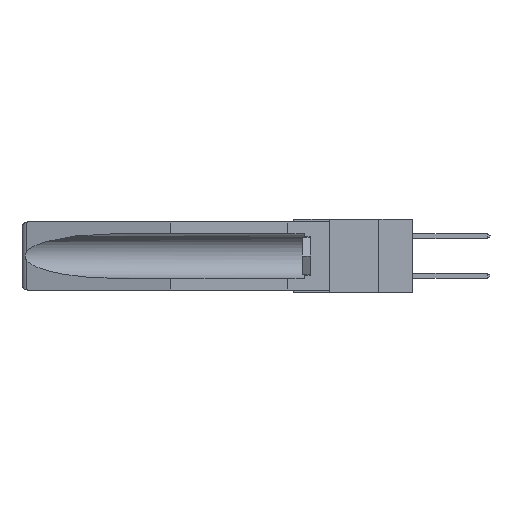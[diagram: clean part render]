
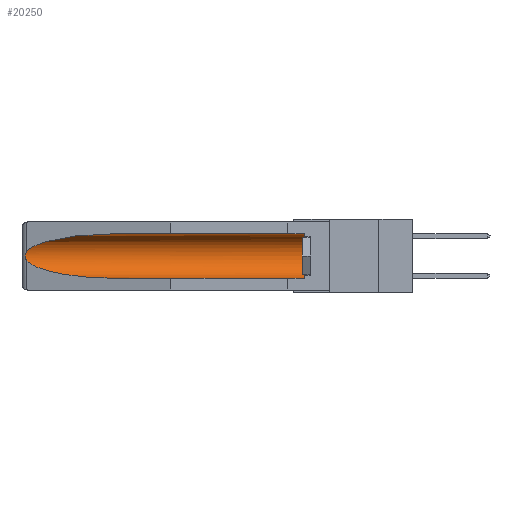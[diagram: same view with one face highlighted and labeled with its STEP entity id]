
A CAD part, left-side view. The second image highlights one B-rep face of the part: STEP entity #20250.
In plain terms, the highlighted cylindrical face has radius 2.857 mm (diameter 5.715 mm), a partial arc.
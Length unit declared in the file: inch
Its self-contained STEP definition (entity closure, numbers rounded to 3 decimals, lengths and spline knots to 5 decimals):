
#826 = CARTESIAN_POINT ( 'NONE',  ( 0.26537, 1.52718, -0.14972 ) ) ;
#1034 = CARTESIAN_POINT ( 'NONE',  ( 0.155, 1.07973, -0.059 ) ) ;
#1538 = ORIENTED_EDGE ( 'NONE', *, *, #7054, .T. ) ;
#2499 = CARTESIAN_POINT ( 'NONE',  ( 0.2673, 1.5327, -0.16383 ) ) ;
#2968 = CARTESIAN_POINT ( 'NONE',  ( 0.155, 1.07973, -0.284 ) ) ;
#3043 = CARTESIAN_POINT ( 'NONE',  ( 0.26655, 1.53094, -0.18657 ) ) ;
#3366 = CARTESIAN_POINT ( 'NONE',  ( 0.155, 0.126, -0.284 ) ) ;
#3527 = VECTOR ( 'NONE', #13411, 39.37008 ) ;
#3944 = VERTEX_POINT ( 'NONE', #24276 ) ;
#4570 = ORIENTED_EDGE ( 'NONE', *, *, #11804, .T. ) ;
#4957 = VERTEX_POINT ( 'NONE', #2968 ) ;
#5781 = CARTESIAN_POINT ( 'NONE',  ( 0.155, -0.30754, -0.059 ) ) ;
#5814 = CARTESIAN_POINT ( 'NONE',  ( 0.2675, 1.53308, -0.17534 ) ) ;
#6683 = VERTEX_POINT ( 'NONE', #3366 ) ;
#6965 = AXIS2_PLACEMENT_3D ( 'NONE', #26146, #28733, #7916 ) ;
#7054 = EDGE_CURVE ( 'NONE', #29487, #24062, #8489, .T. ) ;
#7558 = CYLINDRICAL_SURFACE ( 'NONE', #6965, 0.1125 ) ;
#7916 = DIRECTION ( 'NONE',  ( 0., 0., 1. ) ) ;
#8083 = CARTESIAN_POINT ( 'NONE',  ( 0.26537, 1.52718, -0.19328 ) ) ;
#8441 = CARTESIAN_POINT ( 'NONE',  ( 0.21114, 1.30732, -0.059 ) ) ;
#8489 = B_SPLINE_CURVE_WITH_KNOTS ( 'NONE', 3,
 ( #28002, #10545, #10204, #2499, #30851, #5814, #18343, #3043, #13470, #8083 ),
 .UNSPECIFIED., .F., .F.,
 ( 4, 2, 2, 2, 4 ),
 ( 0., 0.00029, 0.00058, 0.00087, 0.00117 ),
 .UNSPECIFIED. ) ;
#8607 = CARTESIAN_POINT ( 'NONE',  ( 0.25451, 1.48313, -0.24835 ) ) ;
#9104 = CARTESIAN_POINT ( 'NONE',  ( 0.26537, 1.52718, -0.14972 ) ) ;
#9569 = FACE_OUTER_BOUND ( 'NONE', #10806, .T. ) ;
#10052 = AXIS2_PLACEMENT_3D ( 'NONE', #29428, #29658, #29765 ) ;
#10204 = CARTESIAN_POINT ( 'NONE',  ( 0.26654, 1.53092, -0.15636 ) ) ;
#10545 = CARTESIAN_POINT ( 'NONE',  ( 0.26597, 1.52961, -0.15275 ) ) ;
#10806 = EDGE_LOOP ( 'NONE', ( #16528, #1538, #20904, #32389, #29217, #4570 ) ) ;
#11098 = VERTEX_POINT ( 'NONE', #21315 ) ;
#11293 = CARTESIAN_POINT ( 'NONE',  ( 0.26537, 1.52718, -0.19328 ) ) ;
#11804 = EDGE_CURVE ( 'NONE', #11098, #3944, #29886, .T. ) ;
#13411 = DIRECTION ( 'NONE',  ( 0., 1., 0. ) ) ;
#13470 = CARTESIAN_POINT ( 'NONE',  ( 0.26597, 1.5296, -0.19026 ) ) ;
#13874 = CARTESIAN_POINT ( 'NONE',  ( 0.155, 1.07973, -0.284 ) ) ;
#16363 = CARTESIAN_POINT ( 'NONE',  ( 0.25451, 1.48313, -0.09465 ) ) ;
#16528 = ORIENTED_EDGE ( 'NONE', *, *, #18976, .T. ) ;
#17099 = CIRCLE ( 'NONE', #10052, 0.1125 ) ;
#18212 = VECTOR ( 'NONE', #19312, 39.37008 ) ;
#18343 = CARTESIAN_POINT ( 'NONE',  ( 0.2673, 1.53269, -0.17917 ) ) ;
#18976 = EDGE_CURVE ( 'NONE', #3944, #29487, #24719, .T. ) ;
#19312 = DIRECTION ( 'NONE',  ( 0., 1., 0. ) ) ;
#20250 = ADVANCED_FACE ( 'NONE', ( #9569 ), #7558, .F. ) ;
#20904 = ORIENTED_EDGE ( 'NONE', *, *, #21746, .T. ) ;
#21315 = CARTESIAN_POINT ( 'NONE',  ( 0.155, 0.126, -0.059 ) ) ;
#21432 = CARTESIAN_POINT ( 'NONE',  ( 0.21114, 1.30732, -0.284 ) ) ;
#21746 = EDGE_CURVE ( 'NONE', #24062, #4957, #25312, .T. ) ;
#24062 = VERTEX_POINT ( 'NONE', #33067 ) ;
#24276 = CARTESIAN_POINT ( 'NONE',  ( 0.155, 1.07973, -0.059 ) ) ;
#24719 =( BOUNDED_CURVE ( )  B_SPLINE_CURVE ( 3, ( #1034, #8441, #16363, #826 ),
 .UNSPECIFIED., .F., .F. ) 
 B_SPLINE_CURVE_WITH_KNOTS ( ( 4, 4 ),
 ( 4.71239, 6.08839 ),
 .UNSPECIFIED. ) 
 CURVE ( )  GEOMETRIC_REPRESENTATION_ITEM ( )  RATIONAL_B_SPLINE_CURVE ( ( 1., 0.848, 0.848, 1. ) ) 
 REPRESENTATION_ITEM ( '' )  );
#25312 =( BOUNDED_CURVE ( )  B_SPLINE_CURVE ( 3, ( #11293, #8607, #21432, #13874 ),
 .UNSPECIFIED., .F., .F. ) 
 B_SPLINE_CURVE_WITH_KNOTS ( ( 4, 4 ),
 ( 0.1948, 1.5708 ),
 .UNSPECIFIED. ) 
 CURVE ( )  GEOMETRIC_REPRESENTATION_ITEM ( )  RATIONAL_B_SPLINE_CURVE ( ( 1., 0.848, 0.848, 1. ) ) 
 REPRESENTATION_ITEM ( '' )  );
#26088 = EDGE_CURVE ( 'NONE', #6683, #4957, #28785, .T. ) ;
#26146 = CARTESIAN_POINT ( 'NONE',  ( 0.155, -0.30754, -0.1715 ) ) ;
#26531 = EDGE_CURVE ( 'NONE', #6683, #11098, #17099, .T. ) ;
#28002 = CARTESIAN_POINT ( 'NONE',  ( 0.26537, 1.52718, -0.14972 ) ) ;
#28165 = CARTESIAN_POINT ( 'NONE',  ( 0.155, -0.30754, -0.284 ) ) ;
#28733 = DIRECTION ( 'NONE',  ( 0., 1., 0. ) ) ;
#28785 = LINE ( 'NONE', #28165, #3527 ) ;
#29217 = ORIENTED_EDGE ( 'NONE', *, *, #26531, .T. ) ;
#29428 = CARTESIAN_POINT ( 'NONE',  ( 0.155, 0.126, -0.1715 ) ) ;
#29487 = VERTEX_POINT ( 'NONE', #9104 ) ;
#29658 = DIRECTION ( 'NONE',  ( 0., -1., 0. ) ) ;
#29765 = DIRECTION ( 'NONE',  ( 0., 0., 1. ) ) ;
#29886 = LINE ( 'NONE', #5781, #18212 ) ;
#30851 = CARTESIAN_POINT ( 'NONE',  ( 0.2675, 1.53308, -0.16763 ) ) ;
#32389 = ORIENTED_EDGE ( 'NONE', *, *, #26088, .F. ) ;
#33067 = CARTESIAN_POINT ( 'NONE',  ( 0.26537, 1.52718, -0.19328 ) ) ;
